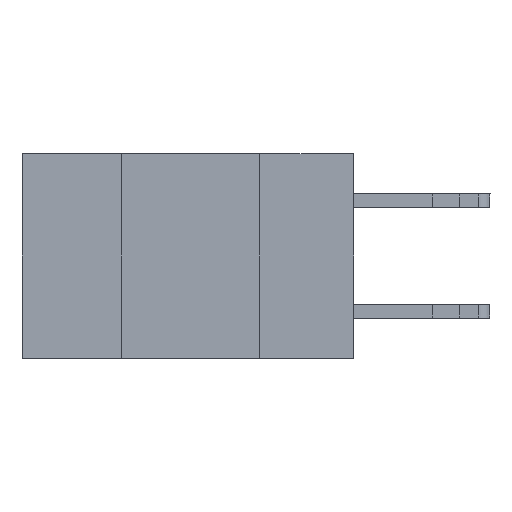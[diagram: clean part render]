
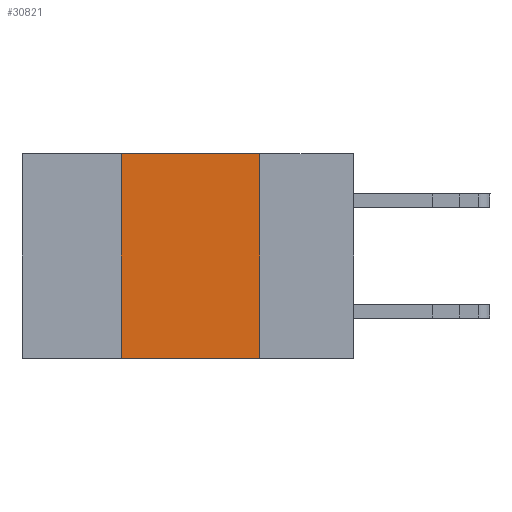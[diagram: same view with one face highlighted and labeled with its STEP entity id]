
A CAD part, left-side view. The second image highlights one B-rep face of the part: STEP entity #30821.
In plain terms, the highlighted planar face has unit normal (-1, 0, 0).
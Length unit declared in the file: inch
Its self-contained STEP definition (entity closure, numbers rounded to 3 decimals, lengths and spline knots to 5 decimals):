
#280 = VECTOR ( 'NONE', #9516, 39.37008 ) ;
#1021 = CARTESIAN_POINT ( 'NONE',  ( 0., 0.6, 0. ) ) ;
#2611 = LINE ( 'NONE', #9856, #33448 ) ;
#4225 = VECTOR ( 'NONE', #5112, 39.37008 ) ;
#4368 = EDGE_CURVE ( 'NONE', #6992, #18947, #12073, .T. ) ;
#5112 = DIRECTION ( 'NONE',  ( 0., 0., 1. ) ) ;
#6022 = CARTESIAN_POINT ( 'NONE',  ( 0., 0.6, 0. ) ) ;
#6992 = VERTEX_POINT ( 'NONE', #28100 ) ;
#7991 = EDGE_CURVE ( 'NONE', #6992, #12877, #2611, .T. ) ;
#8460 = CARTESIAN_POINT ( 'NONE',  ( 0., 0.42, 0. ) ) ;
#9516 = DIRECTION ( 'NONE',  ( 0., -1., 0. ) ) ;
#9856 = CARTESIAN_POINT ( 'NONE',  ( 0., 0.6, -0.37 ) ) ;
#10095 = LINE ( 'NONE', #10641, #13779 ) ;
#10641 = CARTESIAN_POINT ( 'NONE',  ( 0., 0.17, 0. ) ) ;
#11938 = PLANE ( 'NONE',  #17610 ) ;
#12073 = LINE ( 'NONE', #8460, #4225 ) ;
#12200 = EDGE_CURVE ( 'NONE', #27922, #12877, #10095, .T. ) ;
#12877 = VERTEX_POINT ( 'NONE', #17661 ) ;
#13779 = VECTOR ( 'NONE', #14090, 39.37008 ) ;
#13947 = ORIENTED_EDGE ( 'NONE', *, *, #7991, .T. ) ;
#14090 = DIRECTION ( 'NONE',  ( 0., 0., -1. ) ) ;
#14352 = EDGE_LOOP ( 'NONE', ( #30323, #19214, #25931, #13947 ) ) ;
#16022 = DIRECTION ( 'NONE',  ( 0., -1., 0. ) ) ;
#17610 = AXIS2_PLACEMENT_3D ( 'NONE', #6022, #35865, #18208 ) ;
#17661 = CARTESIAN_POINT ( 'NONE',  ( 0., 0.17, -0.37 ) ) ;
#18208 = DIRECTION ( 'NONE',  ( 0., 0., -1. ) ) ;
#18947 = VERTEX_POINT ( 'NONE', #29401 ) ;
#19214 = ORIENTED_EDGE ( 'NONE', *, *, #20941, .F. ) ;
#20941 = EDGE_CURVE ( 'NONE', #18947, #27922, #23751, .T. ) ;
#21083 = FACE_OUTER_BOUND ( 'NONE', #14352, .T. ) ;
#23751 = LINE ( 'NONE', #1021, #280 ) ;
#25931 = ORIENTED_EDGE ( 'NONE', *, *, #4368, .F. ) ;
#27922 = VERTEX_POINT ( 'NONE', #37001 ) ;
#28100 = CARTESIAN_POINT ( 'NONE',  ( 0., 0.42, -0.37 ) ) ;
#29401 = CARTESIAN_POINT ( 'NONE',  ( 0., 0.42, 0. ) ) ;
#30323 = ORIENTED_EDGE ( 'NONE', *, *, #12200, .F. ) ;
#30821 = ADVANCED_FACE ( 'NONE', ( #21083 ), #11938, .F. ) ;
#33448 = VECTOR ( 'NONE', #16022, 39.37008 ) ;
#35865 = DIRECTION ( 'NONE',  ( 1., 0., 0. ) ) ;
#37001 = CARTESIAN_POINT ( 'NONE',  ( 0., 0.17, 0. ) ) ;
